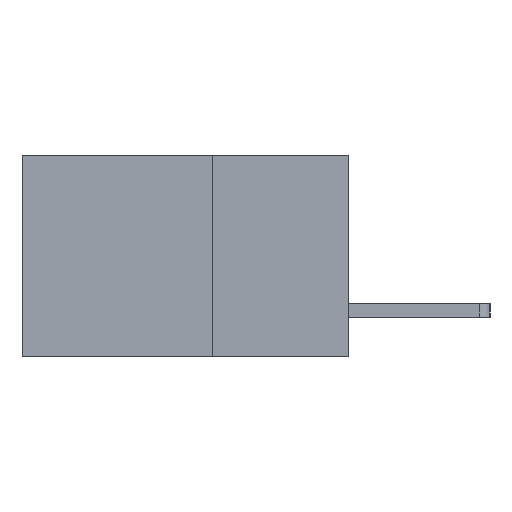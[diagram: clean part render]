
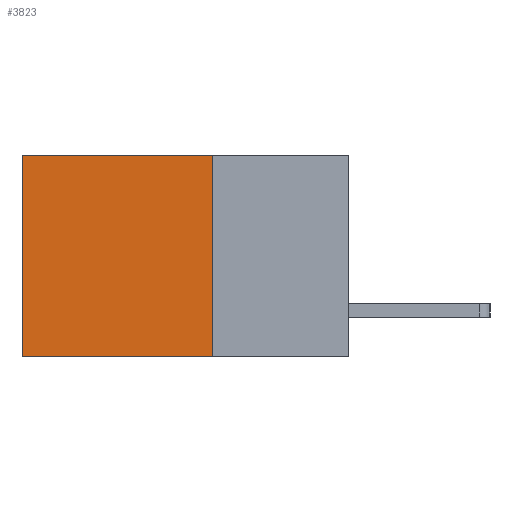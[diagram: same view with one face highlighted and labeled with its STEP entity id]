
A CAD part, left-side view. The second image highlights one B-rep face of the part: STEP entity #3823.
In plain terms, the highlighted planar face has unit normal (-1, 0, 0).
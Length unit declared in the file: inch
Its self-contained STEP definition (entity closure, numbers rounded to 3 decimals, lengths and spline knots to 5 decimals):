
#32 = ORIENTED_EDGE ( 'NONE', *, *, #8183, .T. ) ;
#342 = LINE ( 'NONE', #4122, #4117 ) ;
#945 = LINE ( 'NONE', #7998, #2700 ) ;
#1128 = DIRECTION ( 'NONE',  ( 0., 1., 0. ) ) ;
#1239 = EDGE_CURVE ( 'NONE', #9229, #1616, #945, .T. ) ;
#1358 = AXIS2_PLACEMENT_3D ( 'NONE', #8743, #7320, #8121 ) ;
#1393 = VERTEX_POINT ( 'NONE', #7480 ) ;
#1396 = CARTESIAN_POINT ( 'NONE',  ( 0.298, 0.25, -0.37 ) ) ;
#1445 = EDGE_CURVE ( 'NONE', #1616, #1393, #5293, .T. ) ;
#1575 = VECTOR ( 'NONE', #9202, 39.37008 ) ;
#1616 = VERTEX_POINT ( 'NONE', #4543 ) ;
#2700 = VECTOR ( 'NONE', #4782, 39.37008 ) ;
#2820 = CARTESIAN_POINT ( 'NONE',  ( 0.298, 0.6, 0. ) ) ;
#3000 = ORIENTED_EDGE ( 'NONE', *, *, #1445, .F. ) ;
#3067 = VECTOR ( 'NONE', #7222, 39.37008 ) ;
#3451 = FACE_OUTER_BOUND ( 'NONE', #4679, .T. ) ;
#3810 = LINE ( 'NONE', #6986, #1575 ) ;
#3823 = ADVANCED_FACE ( 'NONE', ( #3451 ), #8971, .F. ) ;
#4117 = VECTOR ( 'NONE', #1128, 39.37008 ) ;
#4122 = CARTESIAN_POINT ( 'NONE',  ( 0.298, 0.25, 0. ) ) ;
#4543 = CARTESIAN_POINT ( 'NONE',  ( 0.298, 0.25, -0.37 ) ) ;
#4679 = EDGE_LOOP ( 'NONE', ( #32, #3000, #5782, #7428 ) ) ;
#4782 = DIRECTION ( 'NONE',  ( 0., 0., -1. ) ) ;
#5293 = LINE ( 'NONE', #1396, #3067 ) ;
#5782 = ORIENTED_EDGE ( 'NONE', *, *, #1239, .F. ) ;
#6986 = CARTESIAN_POINT ( 'NONE',  ( 0.298, 0.6, 0. ) ) ;
#7222 = DIRECTION ( 'NONE',  ( 0., 1., 0. ) ) ;
#7320 = DIRECTION ( 'NONE',  ( 1., 0., 0. ) ) ;
#7428 = ORIENTED_EDGE ( 'NONE', *, *, #8946, .T. ) ;
#7480 = CARTESIAN_POINT ( 'NONE',  ( 0.298, 0.6, -0.37 ) ) ;
#7998 = CARTESIAN_POINT ( 'NONE',  ( 0.298, 0.25, 0. ) ) ;
#8121 = DIRECTION ( 'NONE',  ( 0., 0., -1. ) ) ;
#8183 = EDGE_CURVE ( 'NONE', #8479, #1393, #3810, .T. ) ;
#8479 = VERTEX_POINT ( 'NONE', #2820 ) ;
#8743 = CARTESIAN_POINT ( 'NONE',  ( 0.298, 0.25, 0. ) ) ;
#8946 = EDGE_CURVE ( 'NONE', #9229, #8479, #342, .T. ) ;
#8971 = PLANE ( 'NONE',  #1358 ) ;
#9202 = DIRECTION ( 'NONE',  ( 0., 0., -1. ) ) ;
#9229 = VERTEX_POINT ( 'NONE', #9659 ) ;
#9659 = CARTESIAN_POINT ( 'NONE',  ( 0.298, 0.25, 0. ) ) ;
